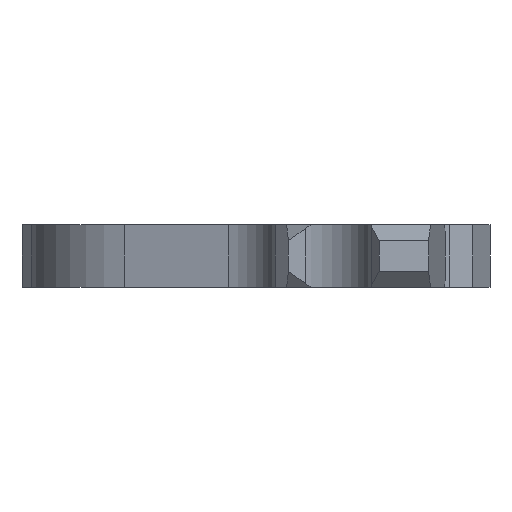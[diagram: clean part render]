
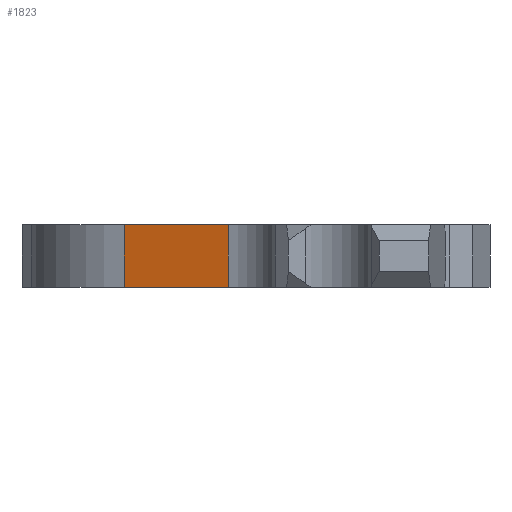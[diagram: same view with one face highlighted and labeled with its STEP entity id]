
A CAD part, left-side view. The second image highlights one B-rep face of the part: STEP entity #1823.
In plain terms, the highlighted planar face has unit normal (-0.958, 0.288, 0).
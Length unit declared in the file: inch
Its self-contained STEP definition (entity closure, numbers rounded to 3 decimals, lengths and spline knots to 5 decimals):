
#142=DIRECTION('',(-0.288,-0.958,0.));
#143=VECTOR('',#142,0.2044);
#144=CARTESIAN_POINT('',(-0.38939,0.51369,
0.11811));
#145=LINE('',#144,#143);
#534=DIRECTION('',(0.288,0.958,0.));
#535=VECTOR('',#534,0.2044);
#536=CARTESIAN_POINT('',(-0.44831,0.31797,0.));
#537=LINE('',#536,#535);
#840=DIRECTION('',(0.,0.,1.));
#841=VECTOR('',#840,0.11811);
#842=CARTESIAN_POINT('',(-0.38939,0.51369,0.));
#843=LINE('',#842,#841);
#847=DIRECTION('',(0.,0.,-1.));
#848=VECTOR('',#847,0.11811);
#849=CARTESIAN_POINT('',(-0.44831,0.31797,
0.11811));
#850=LINE('',#849,#848);
#1117=CARTESIAN_POINT('',(-0.38939,0.51369,
0.11811));
#1118=VERTEX_POINT('',#1117);
#1119=CARTESIAN_POINT('',(-0.44831,0.31797,
0.11811));
#1120=VERTEX_POINT('',#1119);
#1155=CARTESIAN_POINT('',(-0.44831,0.31797,0.));
#1156=VERTEX_POINT('',#1155);
#1157=CARTESIAN_POINT('',(-0.38939,0.51369,0.));
#1158=VERTEX_POINT('',#1157);
#1811=CARTESIAN_POINT('',(-0.38939,0.51369,0.));
#1812=DIRECTION('',(-0.958,0.288,0.));
#1813=DIRECTION('',(-0.288,-0.958,0.));
#1814=AXIS2_PLACEMENT_3D('',#1811,#1812,#1813);
#1815=PLANE('',#1814);
#1816=ORIENTED_EDGE('',*,*,#1502,.T.);
#1817=ORIENTED_EDGE('',*,*,#1806,.T.);
#1818=ORIENTED_EDGE('',*,*,#1326,.T.);
#1820=ORIENTED_EDGE('',*,*,#1819,.T.);
#1821=EDGE_LOOP('',(#1816,#1817,#1818,#1820));
#1822=FACE_OUTER_BOUND('',#1821,.F.);
#1326=EDGE_CURVE('',#1118,#1120,#145,.T.);
#1502=EDGE_CURVE('',#1156,#1158,#537,.T.);
#1806=EDGE_CURVE('',#1158,#1118,#843,.T.);
#1819=EDGE_CURVE('',#1120,#1156,#850,.T.);
#1823=ADVANCED_FACE('',(#1822),#1815,.T.);
